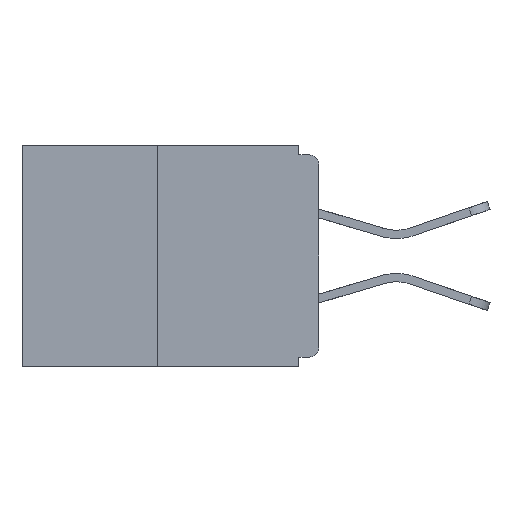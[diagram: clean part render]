
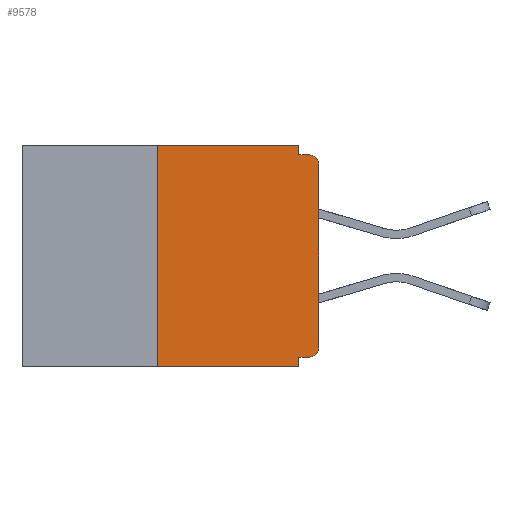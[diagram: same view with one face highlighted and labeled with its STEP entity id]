
A CAD part, left-side view. The second image highlights one B-rep face of the part: STEP entity #9578.
In plain terms, the highlighted planar face has unit normal (-1, 0, 0).
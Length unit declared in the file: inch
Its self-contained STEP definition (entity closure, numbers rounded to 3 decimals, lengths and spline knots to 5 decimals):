
#648 = CARTESIAN_POINT ( 'NONE',  ( 0., 0., -0.03 ) ) ;
#1454 = LINE ( 'NONE', #5887, #12685 ) ;
#1539 = LINE ( 'NONE', #10872, #24670 ) ;
#1612 = VERTEX_POINT ( 'NONE', #20194 ) ;
#1633 = LINE ( 'NONE', #20202, #15664 ) ;
#2422 = CARTESIAN_POINT ( 'NONE',  ( 0., 0.031, -0.015 ) ) ;
#2523 = LINE ( 'NONE', #21389, #8144 ) ;
#3042 = VECTOR ( 'NONE', #12354, 39.37008 ) ;
#3423 = CARTESIAN_POINT ( 'NONE',  ( 0., 0.25, 0. ) ) ;
#3969 = ORIENTED_EDGE ( 'NONE', *, *, #23576, .F. ) ;
#4454 = EDGE_LOOP ( 'NONE', ( #3969, #27888, #11171, #24436, #18566, #28912, #5705, #28493, #18588, #13433 ) ) ;
#4612 = CARTESIAN_POINT ( 'NONE',  ( 0., 0.015, -0.03 ) ) ;
#4939 = DIRECTION ( 'NONE',  ( 0., 0., 1. ) ) ;
#5117 = DIRECTION ( 'NONE',  ( 0., -1., 0. ) ) ;
#5394 = CARTESIAN_POINT ( 'NONE',  ( 0., 0.25, 0. ) ) ;
#5705 = ORIENTED_EDGE ( 'NONE', *, *, #23520, .T. ) ;
#5780 = LINE ( 'NONE', #5394, #19092 ) ;
#5781 = CARTESIAN_POINT ( 'NONE',  ( 0., 0.031, 0. ) ) ;
#5887 = CARTESIAN_POINT ( 'NONE',  ( 0., 0., -0.015 ) ) ;
#7986 = FACE_OUTER_BOUND ( 'NONE', #4454, .T. ) ;
#8144 = VECTOR ( 'NONE', #25181, 39.37008 ) ;
#8760 = CIRCLE ( 'NONE', #14249, 0.015 ) ;
#9578 = ADVANCED_FACE ( 'NONE', ( #7986 ), #10206, .F. ) ;
#9611 = CARTESIAN_POINT ( 'NONE',  ( 0., 0., -0.328 ) ) ;
#10206 = PLANE ( 'NONE',  #18812 ) ;
#10378 = CARTESIAN_POINT ( 'NONE',  ( 0., 0.015, -0.015 ) ) ;
#10872 = CARTESIAN_POINT ( 'NONE',  ( 0., 0.46, -0.343 ) ) ;
#10885 = VERTEX_POINT ( 'NONE', #11287 ) ;
#11171 = ORIENTED_EDGE ( 'NONE', *, *, #19350, .T. ) ;
#11287 = CARTESIAN_POINT ( 'NONE',  ( 0., 0.25, -0.343 ) ) ;
#12354 = DIRECTION ( 'NONE',  ( 0., 1., 0. ) ) ;
#12463 = DIRECTION ( 'NONE',  ( 0., 0., -1. ) ) ;
#12658 = LINE ( 'NONE', #20171, #22447 ) ;
#12685 = VECTOR ( 'NONE', #19190, 39.37008 ) ;
#12854 = LINE ( 'NONE', #9611, #3042 ) ;
#13433 = ORIENTED_EDGE ( 'NONE', *, *, #20349, .F. ) ;
#13711 = CARTESIAN_POINT ( 'NONE',  ( 0., 0., -0.313 ) ) ;
#14090 = CARTESIAN_POINT ( 'NONE',  ( 0., 0.46, 0. ) ) ;
#14249 = AXIS2_PLACEMENT_3D ( 'NONE', #17923, #20165, #17821 ) ;
#14618 = VERTEX_POINT ( 'NONE', #28705 ) ;
#15434 = AXIS2_PLACEMENT_3D ( 'NONE', #4612, #20264, #25250 ) ;
#15664 = VECTOR ( 'NONE', #4939, 39.37008 ) ;
#17154 = CARTESIAN_POINT ( 'NONE',  ( 0., 0.46, 0. ) ) ;
#17596 = EDGE_CURVE ( 'NONE', #1612, #18150, #8760, .T. ) ;
#17821 = DIRECTION ( 'NONE',  ( 0., 0., -1. ) ) ;
#17923 = CARTESIAN_POINT ( 'NONE',  ( 0., 0.015, -0.313 ) ) ;
#18150 = VERTEX_POINT ( 'NONE', #13711 ) ;
#18566 = ORIENTED_EDGE ( 'NONE', *, *, #26304, .F. ) ;
#18588 = ORIENTED_EDGE ( 'NONE', *, *, #20697, .F. ) ;
#18812 = AXIS2_PLACEMENT_3D ( 'NONE', #17154, #19406, #12463 ) ;
#19092 = VECTOR ( 'NONE', #21021, 39.37008 ) ;
#19190 = DIRECTION ( 'NONE',  ( 0., -1., 0. ) ) ;
#19350 = EDGE_CURVE ( 'NONE', #10885, #24367, #1539, .T. ) ;
#19406 = DIRECTION ( 'NONE',  ( 1., 0., 0. ) ) ;
#19558 = EDGE_CURVE ( 'NONE', #20005, #26704, #20787, .T. ) ;
#20005 = VERTEX_POINT ( 'NONE', #648 ) ;
#20165 = DIRECTION ( 'NONE',  ( -1., 0., 0. ) ) ;
#20171 = CARTESIAN_POINT ( 'NONE',  ( 0., 0.031, -0.343 ) ) ;
#20194 = CARTESIAN_POINT ( 'NONE',  ( 0., 0.015, -0.328 ) ) ;
#20202 = CARTESIAN_POINT ( 'NONE',  ( 0., 0., 0. ) ) ;
#20264 = DIRECTION ( 'NONE',  ( -1., 0., 0. ) ) ;
#20349 = EDGE_CURVE ( 'NONE', #23799, #25705, #2523, .T. ) ;
#20697 = EDGE_CURVE ( 'NONE', #25705, #26704, #1454, .T. ) ;
#20787 = CIRCLE ( 'NONE', #15434, 0.015 ) ;
#20984 = EDGE_CURVE ( 'NONE', #14618, #24367, #12658, .T. ) ;
#21021 = DIRECTION ( 'NONE',  ( 0., 0., 1. ) ) ;
#21389 = CARTESIAN_POINT ( 'NONE',  ( 0., 0.031, 0. ) ) ;
#22447 = VECTOR ( 'NONE', #27121, 39.37008 ) ;
#23520 = EDGE_CURVE ( 'NONE', #18150, #20005, #1633, .T. ) ;
#23576 = EDGE_CURVE ( 'NONE', #27828, #23799, #26893, .T. ) ;
#23582 = CARTESIAN_POINT ( 'NONE',  ( 0., 0.031, -0.343 ) ) ;
#23799 = VERTEX_POINT ( 'NONE', #5781 ) ;
#24367 = VERTEX_POINT ( 'NONE', #23582 ) ;
#24436 = ORIENTED_EDGE ( 'NONE', *, *, #20984, .F. ) ;
#24670 = VECTOR ( 'NONE', #28878, 39.37008 ) ;
#24743 = EDGE_CURVE ( 'NONE', #10885, #27828, #5780, .T. ) ;
#25181 = DIRECTION ( 'NONE',  ( 0., 0., -1. ) ) ;
#25250 = DIRECTION ( 'NONE',  ( 0., 0., -1. ) ) ;
#25705 = VERTEX_POINT ( 'NONE', #2422 ) ;
#26304 = EDGE_CURVE ( 'NONE', #1612, #14618, #12854, .T. ) ;
#26704 = VERTEX_POINT ( 'NONE', #10378 ) ;
#26893 = LINE ( 'NONE', #14090, #27254 ) ;
#27121 = DIRECTION ( 'NONE',  ( 0., 0., -1. ) ) ;
#27254 = VECTOR ( 'NONE', #5117, 39.37008 ) ;
#27828 = VERTEX_POINT ( 'NONE', #3423 ) ;
#27888 = ORIENTED_EDGE ( 'NONE', *, *, #24743, .F. ) ;
#28493 = ORIENTED_EDGE ( 'NONE', *, *, #19558, .T. ) ;
#28705 = CARTESIAN_POINT ( 'NONE',  ( 0., 0.031, -0.328 ) ) ;
#28878 = DIRECTION ( 'NONE',  ( 0., -1., 0. ) ) ;
#28912 = ORIENTED_EDGE ( 'NONE', *, *, #17596, .T. ) ;
